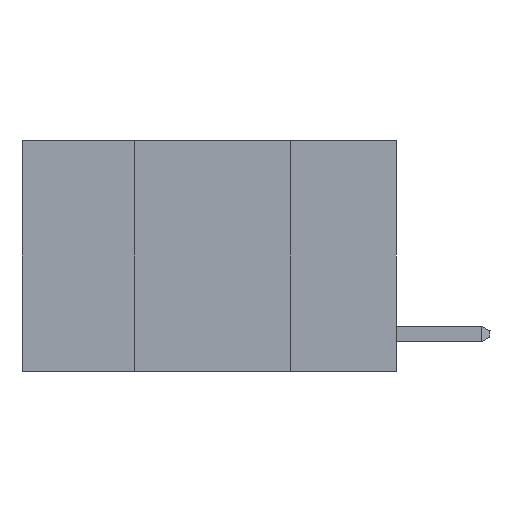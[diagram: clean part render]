
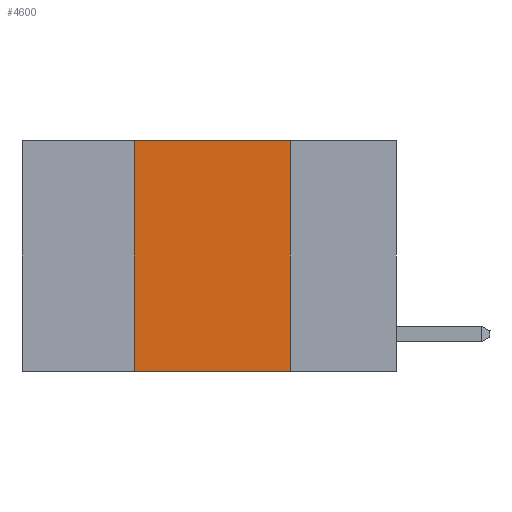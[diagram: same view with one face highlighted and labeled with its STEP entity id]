
A CAD part, left-side view. The second image highlights one B-rep face of the part: STEP entity #4600.
In plain terms, the highlighted planar face has unit normal (-1, 0, 0).
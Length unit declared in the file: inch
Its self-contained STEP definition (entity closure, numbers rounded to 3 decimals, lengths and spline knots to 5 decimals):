
#150 = ORIENTED_EDGE ( 'NONE', *, *, #9860, .T. ) ;
#420 = CARTESIAN_POINT ( 'NONE',  ( 0., 0.6, -0.37 ) ) ;
#705 = VERTEX_POINT ( 'NONE', #3604 ) ;
#1174 = CARTESIAN_POINT ( 'NONE',  ( 0., 0.17, 0. ) ) ;
#1424 = ORIENTED_EDGE ( 'NONE', *, *, #10061, .F. ) ;
#1742 = FACE_OUTER_BOUND ( 'NONE', #10225, .T. ) ;
#2502 = CARTESIAN_POINT ( 'NONE',  ( 0., 0.42, -0.37 ) ) ;
#3169 = CARTESIAN_POINT ( 'NONE',  ( 0., 0.6, 0. ) ) ;
#3604 = CARTESIAN_POINT ( 'NONE',  ( 0., 0.17, -0.37 ) ) ;
#3902 = CARTESIAN_POINT ( 'NONE',  ( 0., 0.42, 0. ) ) ;
#3953 = PLANE ( 'NONE',  #6686 ) ;
#4600 = ADVANCED_FACE ( 'NONE', ( #1742 ), #3953, .F. ) ;
#4880 = VECTOR ( 'NONE', #9085, 39.37008 ) ;
#5130 = DIRECTION ( 'NONE',  ( 0., 0., 1. ) ) ;
#6343 = DIRECTION ( 'NONE',  ( 1., 0., 0. ) ) ;
#6686 = AXIS2_PLACEMENT_3D ( 'NONE', #11277, #6343, #12580 ) ;
#7020 = VERTEX_POINT ( 'NONE', #13451 ) ;
#9085 = DIRECTION ( 'NONE',  ( 0., -1., 0. ) ) ;
#9421 = DIRECTION ( 'NONE',  ( 0., -1., 0. ) ) ;
#9860 = EDGE_CURVE ( 'NONE', #12484, #705, #12412, .T. ) ;
#10061 = EDGE_CURVE ( 'NONE', #7020, #705, #12006, .T. ) ;
#10225 = EDGE_LOOP ( 'NONE', ( #1424, #15619, #14489, #150 ) ) ;
#10706 = LINE ( 'NONE', #3902, #11291 ) ;
#10960 = DIRECTION ( 'NONE',  ( 0., 0., -1. ) ) ;
#10968 = EDGE_CURVE ( 'NONE', #11350, #7020, #11020, .T. ) ;
#11020 = LINE ( 'NONE', #3169, #15842 ) ;
#11277 = CARTESIAN_POINT ( 'NONE',  ( 0., 0.6, 0. ) ) ;
#11291 = VECTOR ( 'NONE', #5130, 39.37008 ) ;
#11350 = VERTEX_POINT ( 'NONE', #12118 ) ;
#12006 = LINE ( 'NONE', #1174, #14161 ) ;
#12118 = CARTESIAN_POINT ( 'NONE',  ( 0., 0.42, 0. ) ) ;
#12412 = LINE ( 'NONE', #420, #4880 ) ;
#12484 = VERTEX_POINT ( 'NONE', #2502 ) ;
#12580 = DIRECTION ( 'NONE',  ( 0., 0., -1. ) ) ;
#13451 = CARTESIAN_POINT ( 'NONE',  ( 0., 0.17, 0. ) ) ;
#14161 = VECTOR ( 'NONE', #10960, 39.37008 ) ;
#14489 = ORIENTED_EDGE ( 'NONE', *, *, #15688, .F. ) ;
#15619 = ORIENTED_EDGE ( 'NONE', *, *, #10968, .F. ) ;
#15688 = EDGE_CURVE ( 'NONE', #12484, #11350, #10706, .T. ) ;
#15842 = VECTOR ( 'NONE', #9421, 39.37008 ) ;
